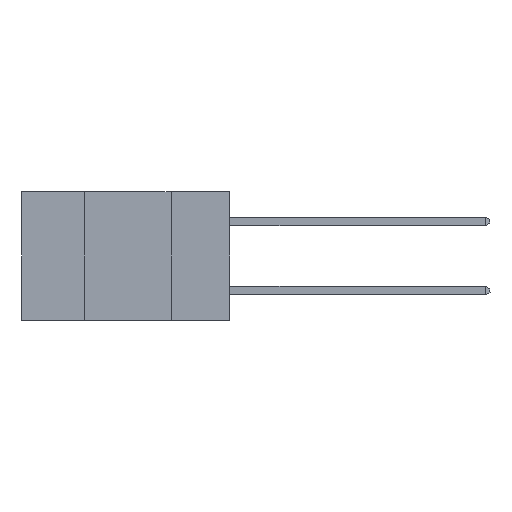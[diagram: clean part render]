
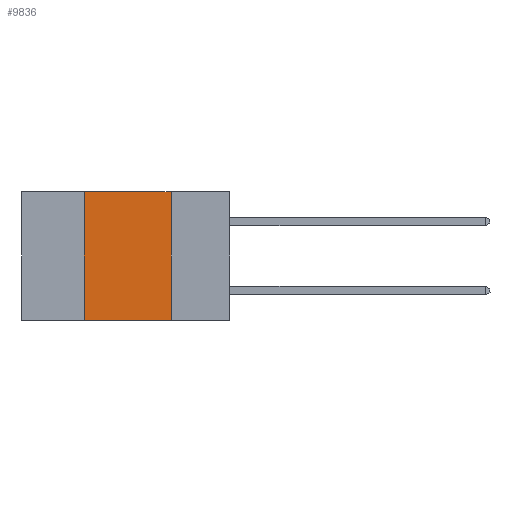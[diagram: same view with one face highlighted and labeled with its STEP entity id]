
A CAD part, left-side view. The second image highlights one B-rep face of the part: STEP entity #9836.
In plain terms, the highlighted planar face has unit normal (-1, 0, 0).
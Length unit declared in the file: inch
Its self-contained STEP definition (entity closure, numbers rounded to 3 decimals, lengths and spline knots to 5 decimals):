
#2562 = CARTESIAN_POINT ( 'NONE',  ( 0., 0.42, -0.37 ) ) ;
#2829 = CARTESIAN_POINT ( 'NONE',  ( 0., 0.17, 0. ) ) ;
#2958 = EDGE_LOOP ( 'NONE', ( #13354, #8720, #22289, #28902 ) ) ;
#4294 = CARTESIAN_POINT ( 'NONE',  ( 0., 0.6, -0.37 ) ) ;
#4786 = CARTESIAN_POINT ( 'NONE',  ( 0., 0.17, 0. ) ) ;
#5050 = CARTESIAN_POINT ( 'NONE',  ( 0., 0.6, 0. ) ) ;
#5998 = LINE ( 'NONE', #4294, #29923 ) ;
#6468 = PLANE ( 'NONE',  #9357 ) ;
#8720 = ORIENTED_EDGE ( 'NONE', *, *, #21845, .F. ) ;
#9009 = VECTOR ( 'NONE', #9705, 39.37008 ) ;
#9357 = AXIS2_PLACEMENT_3D ( 'NONE', #24619, #29480, #29570 ) ;
#9438 = DIRECTION ( 'NONE',  ( 0., 0., -1. ) ) ;
#9705 = DIRECTION ( 'NONE',  ( 0., -1., 0. ) ) ;
#9836 = ADVANCED_FACE ( 'NONE', ( #23822 ), #6468, .F. ) ;
#13354 = ORIENTED_EDGE ( 'NONE', *, *, #22318, .F. ) ;
#16581 = LINE ( 'NONE', #4786, #25271 ) ;
#16741 = VERTEX_POINT ( 'NONE', #22410 ) ;
#17368 = CARTESIAN_POINT ( 'NONE',  ( 0., 0.42, 0. ) ) ;
#18776 = DIRECTION ( 'NONE',  ( 0., 0., 1. ) ) ;
#18930 = LINE ( 'NONE', #23244, #26849 ) ;
#20281 = DIRECTION ( 'NONE',  ( 0., -1., 0. ) ) ;
#21808 = VERTEX_POINT ( 'NONE', #2829 ) ;
#21845 = EDGE_CURVE ( 'NONE', #24620, #21808, #22418, .T. ) ;
#22289 = ORIENTED_EDGE ( 'NONE', *, *, #27824, .F. ) ;
#22318 = EDGE_CURVE ( 'NONE', #21808, #16741, #16581, .T. ) ;
#22410 = CARTESIAN_POINT ( 'NONE',  ( 0., 0.17, -0.37 ) ) ;
#22418 = LINE ( 'NONE', #5050, #9009 ) ;
#23244 = CARTESIAN_POINT ( 'NONE',  ( 0., 0.42, 0. ) ) ;
#23822 = FACE_OUTER_BOUND ( 'NONE', #2958, .T. ) ;
#24619 = CARTESIAN_POINT ( 'NONE',  ( 0., 0.6, 0. ) ) ;
#24620 = VERTEX_POINT ( 'NONE', #17368 ) ;
#24903 = VERTEX_POINT ( 'NONE', #2562 ) ;
#25271 = VECTOR ( 'NONE', #9438, 39.37008 ) ;
#25558 = EDGE_CURVE ( 'NONE', #24903, #16741, #5998, .T. ) ;
#26849 = VECTOR ( 'NONE', #18776, 39.37008 ) ;
#27824 = EDGE_CURVE ( 'NONE', #24903, #24620, #18930, .T. ) ;
#28902 = ORIENTED_EDGE ( 'NONE', *, *, #25558, .T. ) ;
#29480 = DIRECTION ( 'NONE',  ( 1., 0., 0. ) ) ;
#29570 = DIRECTION ( 'NONE',  ( 0., 0., -1. ) ) ;
#29923 = VECTOR ( 'NONE', #20281, 39.37008 ) ;
